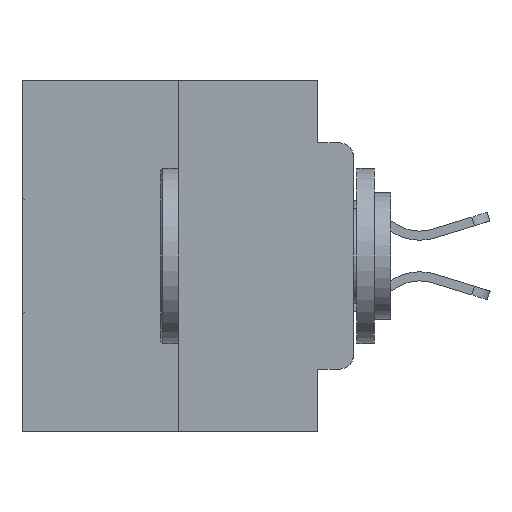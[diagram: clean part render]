
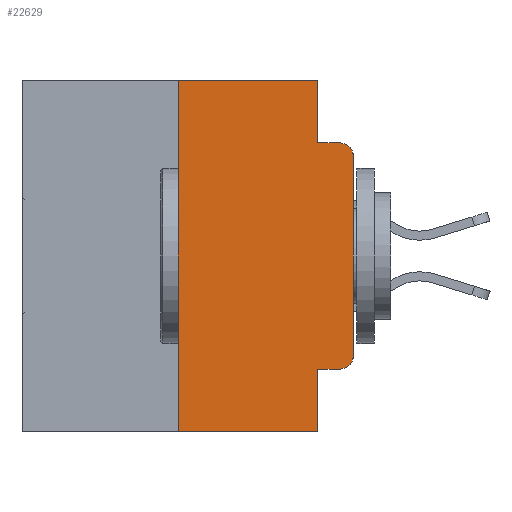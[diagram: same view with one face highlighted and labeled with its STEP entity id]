
A CAD part, left-side view. The second image highlights one B-rep face of the part: STEP entity #22629.
In plain terms, the highlighted planar face has unit normal (-1, 0, 0).
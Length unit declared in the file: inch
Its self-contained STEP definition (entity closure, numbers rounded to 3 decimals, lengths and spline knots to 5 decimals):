
#434 = AXIS2_PLACEMENT_3D ( 'NONE', #28660, #29157, #10620 ) ;
#1094 = CARTESIAN_POINT ( 'NONE',  ( 0., 0.473, 0. ) ) ;
#1352 = CARTESIAN_POINT ( 'NONE',  ( 0., 0.051, -0.5 ) ) ;
#1529 = CARTESIAN_POINT ( 'NONE',  ( 0., 0.051, 0. ) ) ;
#1809 = EDGE_CURVE ( 'NONE', #17384, #21118, #24406, .T. ) ;
#1947 = EDGE_CURVE ( 'NONE', #4093, #10122, #20001, .T. ) ;
#2128 = EDGE_CURVE ( 'NONE', #4955, #17384, #19261, .T. ) ;
#2290 = EDGE_LOOP ( 'NONE', ( #8714, #4705, #3370, #15828, #26637, #14721, #16161, #14238, #27798, #18150 ) ) ;
#2533 = EDGE_CURVE ( 'NONE', #4955, #21923, #22158, .T. ) ;
#2586 = CARTESIAN_POINT ( 'NONE',  ( 0., 0.02, -0.1085 ) ) ;
#2901 = CARTESIAN_POINT ( 'NONE',  ( 0., 0.051, -0.0885 ) ) ;
#3370 = ORIENTED_EDGE ( 'NONE', *, *, #6892, .F. ) ;
#4093 = VERTEX_POINT ( 'NONE', #12627 ) ;
#4205 = EDGE_CURVE ( 'NONE', #4093, #21923, #10103, .T. ) ;
#4462 = VERTEX_POINT ( 'NONE', #7098 ) ;
#4583 = FACE_OUTER_BOUND ( 'NONE', #2290, .T. ) ;
#4705 = ORIENTED_EDGE ( 'NONE', *, *, #27951, .T. ) ;
#4955 = VERTEX_POINT ( 'NONE', #5350 ) ;
#5112 = DIRECTION ( 'NONE',  ( 0., 0., -1. ) ) ;
#5350 = CARTESIAN_POINT ( 'NONE',  ( 0., 0.051, -0.4115 ) ) ;
#5389 = EDGE_CURVE ( 'NONE', #26015, #27926, #9280, .T. ) ;
#5452 = DIRECTION ( 'NONE',  ( 0., 0., -1. ) ) ;
#5506 = EDGE_CURVE ( 'NONE', #21118, #16916, #8167, .T. ) ;
#5669 = VECTOR ( 'NONE', #5112, 39.37008 ) ;
#6892 = EDGE_CURVE ( 'NONE', #27926, #4462, #20282, .T. ) ;
#7097 = VECTOR ( 'NONE', #27733, 39.37008 ) ;
#7098 = CARTESIAN_POINT ( 'NONE',  ( 0., 0.02, -0.0885 ) ) ;
#7940 = VECTOR ( 'NONE', #10092, 39.37008 ) ;
#8102 = CARTESIAN_POINT ( 'NONE',  ( 0., 0.25, 0. ) ) ;
#8142 = CIRCLE ( 'NONE', #27699, 0.02 ) ;
#8167 = LINE ( 'NONE', #20701, #7097 ) ;
#8393 = VECTOR ( 'NONE', #16199, 39.37008 ) ;
#8714 = ORIENTED_EDGE ( 'NONE', *, *, #5506, .T. ) ;
#9280 = LINE ( 'NONE', #23976, #5669 ) ;
#9495 = LINE ( 'NONE', #15337, #21486 ) ;
#10092 = DIRECTION ( 'NONE',  ( 0., -1., 0. ) ) ;
#10103 = LINE ( 'NONE', #26928, #12854 ) ;
#10122 = VERTEX_POINT ( 'NONE', #26673 ) ;
#10185 = CARTESIAN_POINT ( 'NONE',  ( 0., 0.051, 0. ) ) ;
#10427 = DIRECTION ( 'NONE',  ( 0., 0., 1. ) ) ;
#10539 = DIRECTION ( 'NONE',  ( 0., -1., 0. ) ) ;
#10620 = DIRECTION ( 'NONE',  ( 0., 0., -1. ) ) ;
#10728 = DIRECTION ( 'NONE',  ( 0., 0., -1. ) ) ;
#12113 = EDGE_CURVE ( 'NONE', #10122, #26015, #9495, .T. ) ;
#12627 = CARTESIAN_POINT ( 'NONE',  ( 0., 0.25, -0.5 ) ) ;
#12854 = VECTOR ( 'NONE', #10539, 39.37008 ) ;
#13213 = DIRECTION ( 'NONE',  ( 0., -1., 0. ) ) ;
#14238 = ORIENTED_EDGE ( 'NONE', *, *, #2533, .F. ) ;
#14721 = ORIENTED_EDGE ( 'NONE', *, *, #1947, .F. ) ;
#15337 = CARTESIAN_POINT ( 'NONE',  ( 0., 0.473, 0. ) ) ;
#15828 = ORIENTED_EDGE ( 'NONE', *, *, #5389, .F. ) ;
#16161 = ORIENTED_EDGE ( 'NONE', *, *, #4205, .T. ) ;
#16199 = DIRECTION ( 'NONE',  ( 0., -1., 0. ) ) ;
#16733 = VECTOR ( 'NONE', #5452, 39.37008 ) ;
#16916 = VERTEX_POINT ( 'NONE', #25610 ) ;
#17384 = VERTEX_POINT ( 'NONE', #26795 ) ;
#17451 = CARTESIAN_POINT ( 'NONE',  ( 0., 0.051, -0.0885 ) ) ;
#18150 = ORIENTED_EDGE ( 'NONE', *, *, #1809, .T. ) ;
#18806 = DIRECTION ( 'NONE',  ( 0., 0., -1. ) ) ;
#19261 = LINE ( 'NONE', #20598, #8393 ) ;
#20001 = LINE ( 'NONE', #8102, #28416 ) ;
#20282 = LINE ( 'NONE', #2901, #7940 ) ;
#20598 = CARTESIAN_POINT ( 'NONE',  ( 0., 0.051, -0.4115 ) ) ;
#20701 = CARTESIAN_POINT ( 'NONE',  ( 0., 0., 0. ) ) ;
#21118 = VERTEX_POINT ( 'NONE', #28289 ) ;
#21486 = VECTOR ( 'NONE', #13213, 39.37008 ) ;
#21923 = VERTEX_POINT ( 'NONE', #1352 ) ;
#22158 = LINE ( 'NONE', #10185, #16733 ) ;
#22629 = ADVANCED_FACE ( 'NONE', ( #4583 ), #26822, .F. ) ;
#23976 = CARTESIAN_POINT ( 'NONE',  ( 0., 0.051, 0. ) ) ;
#24406 = CIRCLE ( 'NONE', #434, 0.02 ) ;
#25610 = CARTESIAN_POINT ( 'NONE',  ( 0., 0., -0.1085 ) ) ;
#25869 = DIRECTION ( 'NONE',  ( -1., 0., 0. ) ) ;
#26015 = VERTEX_POINT ( 'NONE', #1529 ) ;
#26637 = ORIENTED_EDGE ( 'NONE', *, *, #12113, .F. ) ;
#26673 = CARTESIAN_POINT ( 'NONE',  ( 0., 0.25, 0. ) ) ;
#26795 = CARTESIAN_POINT ( 'NONE',  ( 0., 0.02, -0.4115 ) ) ;
#26822 = PLANE ( 'NONE',  #28609 ) ;
#26928 = CARTESIAN_POINT ( 'NONE',  ( 0., 0.473, -0.5 ) ) ;
#27699 = AXIS2_PLACEMENT_3D ( 'NONE', #2586, #25869, #18806 ) ;
#27733 = DIRECTION ( 'NONE',  ( 0., 0., 1. ) ) ;
#27798 = ORIENTED_EDGE ( 'NONE', *, *, #2128, .T. ) ;
#27926 = VERTEX_POINT ( 'NONE', #17451 ) ;
#27951 = EDGE_CURVE ( 'NONE', #16916, #4462, #8142, .T. ) ;
#28289 = CARTESIAN_POINT ( 'NONE',  ( 0., 0., -0.3915 ) ) ;
#28416 = VECTOR ( 'NONE', #10427, 39.37008 ) ;
#28609 = AXIS2_PLACEMENT_3D ( 'NONE', #1094, #29372, #10728 ) ;
#28660 = CARTESIAN_POINT ( 'NONE',  ( 0., 0.02, -0.3915 ) ) ;
#29157 = DIRECTION ( 'NONE',  ( -1., 0., 0. ) ) ;
#29372 = DIRECTION ( 'NONE',  ( 1., 0., 0. ) ) ;
